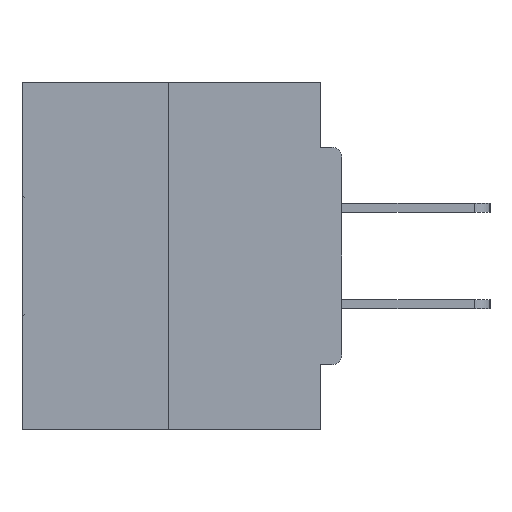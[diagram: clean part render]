
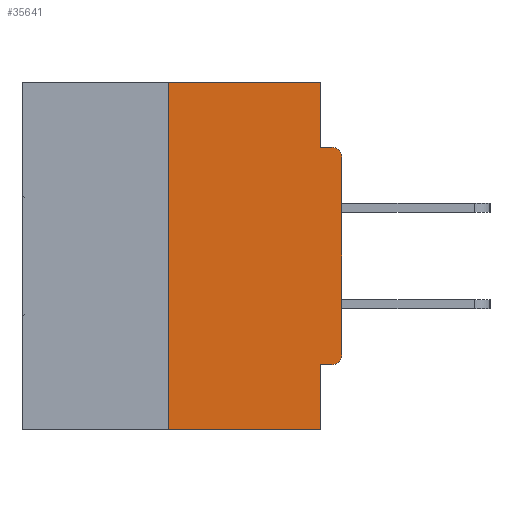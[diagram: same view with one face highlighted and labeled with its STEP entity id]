
A CAD part, left-side view. The second image highlights one B-rep face of the part: STEP entity #35641.
In plain terms, the highlighted planar face has unit normal (-1, 0, 0).
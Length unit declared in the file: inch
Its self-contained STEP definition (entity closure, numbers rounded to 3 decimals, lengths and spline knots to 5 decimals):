
#1261 = EDGE_CURVE ( 'NONE', #26314, #3643, #35673, .T. ) ;
#1411 = VERTEX_POINT ( 'NONE', #27119 ) ;
#2394 = EDGE_CURVE ( 'NONE', #26314, #18412, #6992, .T. ) ;
#2865 = VECTOR ( 'NONE', #5337, 39.37008 ) ;
#3149 = VERTEX_POINT ( 'NONE', #33076 ) ;
#3643 = VERTEX_POINT ( 'NONE', #29270 ) ;
#3707 = ORIENTED_EDGE ( 'NONE', *, *, #2394, .F. ) ;
#3820 = CARTESIAN_POINT ( 'NONE',  ( 0., 0.46, 0. ) ) ;
#3851 = ORIENTED_EDGE ( 'NONE', *, *, #31598, .F. ) ;
#5082 = DIRECTION ( 'NONE',  ( -1., 0., 0. ) ) ;
#5337 = DIRECTION ( 'NONE',  ( 0., -1., 0. ) ) ;
#5859 = EDGE_CURVE ( 'NONE', #39965, #29679, #26435, .T. ) ;
#6730 = PLANE ( 'NONE',  #14141 ) ;
#6930 = CARTESIAN_POINT ( 'NONE',  ( 0., 0.015, -0.4065 ) ) ;
#6982 = EDGE_CURVE ( 'NONE', #10766, #29679, #22324, .T. ) ;
#6992 = LINE ( 'NONE', #25237, #12910 ) ;
#7128 = VECTOR ( 'NONE', #40096, 39.37008 ) ;
#8320 = LINE ( 'NONE', #3820, #29458 ) ;
#8555 = CARTESIAN_POINT ( 'NONE',  ( 0., 0., -0.4065 ) ) ;
#8666 = DIRECTION ( 'NONE',  ( 0., 0., 1. ) ) ;
#8677 = DIRECTION ( 'NONE',  ( 0., 0., -1. ) ) ;
#9390 = CARTESIAN_POINT ( 'NONE',  ( 0., 0.031, -0.0935 ) ) ;
#10016 = DIRECTION ( 'NONE',  ( 0., 0., -1. ) ) ;
#10395 = CARTESIAN_POINT ( 'NONE',  ( 0., 0.031, 0. ) ) ;
#10766 = VERTEX_POINT ( 'NONE', #27957 ) ;
#11048 = AXIS2_PLACEMENT_3D ( 'NONE', #39946, #34098, #19199 ) ;
#11175 = CIRCLE ( 'NONE', #11048, 0.015 ) ;
#11382 = DIRECTION ( 'NONE',  ( 0., 0., -1. ) ) ;
#12109 = CARTESIAN_POINT ( 'NONE',  ( 0., 0.031, 0. ) ) ;
#12589 = VERTEX_POINT ( 'NONE', #6930 ) ;
#12910 = VECTOR ( 'NONE', #31589, 39.37008 ) ;
#13194 = DIRECTION ( 'NONE',  ( 1., 0., 0. ) ) ;
#14141 = AXIS2_PLACEMENT_3D ( 'NONE', #28841, #13194, #10016 ) ;
#15336 = CARTESIAN_POINT ( 'NONE',  ( 0., 0.25, -0.5 ) ) ;
#16249 = ORIENTED_EDGE ( 'NONE', *, *, #22246, .T. ) ;
#17227 = ORIENTED_EDGE ( 'NONE', *, *, #6982, .T. ) ;
#17402 = CARTESIAN_POINT ( 'NONE',  ( 0., 0., 0. ) ) ;
#18412 = VERTEX_POINT ( 'NONE', #21692 ) ;
#19138 = EDGE_CURVE ( 'NONE', #12589, #1411, #11175, .T. ) ;
#19199 = DIRECTION ( 'NONE',  ( 0., 0., -1. ) ) ;
#20738 = VERTEX_POINT ( 'NONE', #10395 ) ;
#21096 = VECTOR ( 'NONE', #8677, 39.37008 ) ;
#21692 = CARTESIAN_POINT ( 'NONE',  ( 0., 0.25, 0. ) ) ;
#22246 = EDGE_CURVE ( 'NONE', #1411, #10766, #36251, .T. ) ;
#22324 = CIRCLE ( 'NONE', #36700, 0.015 ) ;
#22400 = ORIENTED_EDGE ( 'NONE', *, *, #29891, .F. ) ;
#23878 = CARTESIAN_POINT ( 'NONE',  ( 0., 0.015, -0.0935 ) ) ;
#23900 = CARTESIAN_POINT ( 'NONE',  ( 0., 0.015, -0.1085 ) ) ;
#25237 = CARTESIAN_POINT ( 'NONE',  ( 0., 0.25, 0. ) ) ;
#26314 = VERTEX_POINT ( 'NONE', #15336 ) ;
#26435 = LINE ( 'NONE', #27307, #2865 ) ;
#26833 = EDGE_CURVE ( 'NONE', #3149, #3643, #36934, .T. ) ;
#27119 = CARTESIAN_POINT ( 'NONE',  ( 0., 0., -0.3915 ) ) ;
#27307 = CARTESIAN_POINT ( 'NONE',  ( 0., 0., -0.0935 ) ) ;
#27345 = VECTOR ( 'NONE', #8666, 39.37008 ) ;
#27684 = EDGE_CURVE ( 'NONE', #20738, #39965, #38288, .T. ) ;
#27806 = ORIENTED_EDGE ( 'NONE', *, *, #27684, .F. ) ;
#27957 = CARTESIAN_POINT ( 'NONE',  ( 0., 0., -0.1085 ) ) ;
#28015 = VECTOR ( 'NONE', #37184, 39.37008 ) ;
#28512 = ORIENTED_EDGE ( 'NONE', *, *, #5859, .F. ) ;
#28714 = VECTOR ( 'NONE', #32638, 39.37008 ) ;
#28841 = CARTESIAN_POINT ( 'NONE',  ( 0., 0.46, 0. ) ) ;
#29270 = CARTESIAN_POINT ( 'NONE',  ( 0., 0.031, -0.5 ) ) ;
#29458 = VECTOR ( 'NONE', #34953, 39.37008 ) ;
#29679 = VERTEX_POINT ( 'NONE', #23878 ) ;
#29891 = EDGE_CURVE ( 'NONE', #18412, #20738, #8320, .T. ) ;
#30724 = CARTESIAN_POINT ( 'NONE',  ( 0., 0.031, -0.5 ) ) ;
#31589 = DIRECTION ( 'NONE',  ( 0., 0., 1. ) ) ;
#31598 = EDGE_CURVE ( 'NONE', #12589, #3149, #37669, .T. ) ;
#32578 = ORIENTED_EDGE ( 'NONE', *, *, #19138, .T. ) ;
#32638 = DIRECTION ( 'NONE',  ( 0., -1., 0. ) ) ;
#33076 = CARTESIAN_POINT ( 'NONE',  ( 0., 0.031, -0.4065 ) ) ;
#33229 = ORIENTED_EDGE ( 'NONE', *, *, #26833, .F. ) ;
#34098 = DIRECTION ( 'NONE',  ( -1., 0., 0. ) ) ;
#34953 = DIRECTION ( 'NONE',  ( 0., -1., 0. ) ) ;
#35538 = CARTESIAN_POINT ( 'NONE',  ( 0., 0.46, -0.5 ) ) ;
#35641 = ADVANCED_FACE ( 'NONE', ( #37340 ), #6730, .F. ) ;
#35673 = LINE ( 'NONE', #35538, #28714 ) ;
#36251 = LINE ( 'NONE', #17402, #27345 ) ;
#36700 = AXIS2_PLACEMENT_3D ( 'NONE', #23900, #5082, #11382 ) ;
#36934 = LINE ( 'NONE', #30724, #28015 ) ;
#37184 = DIRECTION ( 'NONE',  ( 0., 0., -1. ) ) ;
#37340 = FACE_OUTER_BOUND ( 'NONE', #38100, .T. ) ;
#37669 = LINE ( 'NONE', #8555, #7128 ) ;
#38100 = EDGE_LOOP ( 'NONE', ( #22400, #3707, #40586, #33229, #3851, #32578, #16249, #17227, #28512, #27806 ) ) ;
#38288 = LINE ( 'NONE', #12109, #21096 ) ;
#39946 = CARTESIAN_POINT ( 'NONE',  ( 0., 0.015, -0.3915 ) ) ;
#39965 = VERTEX_POINT ( 'NONE', #9390 ) ;
#40096 = DIRECTION ( 'NONE',  ( 0., 1., 0. ) ) ;
#40586 = ORIENTED_EDGE ( 'NONE', *, *, #1261, .T. ) ;
